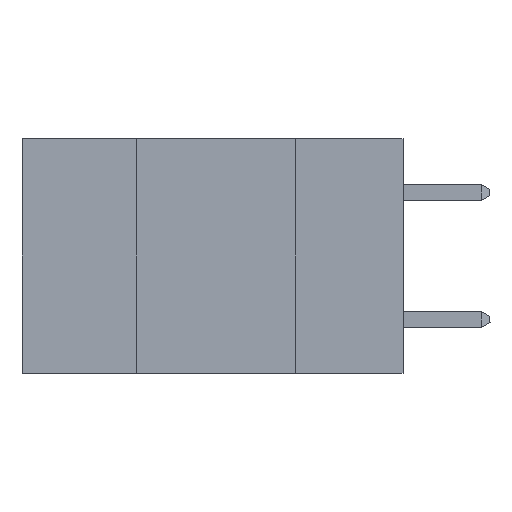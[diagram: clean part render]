
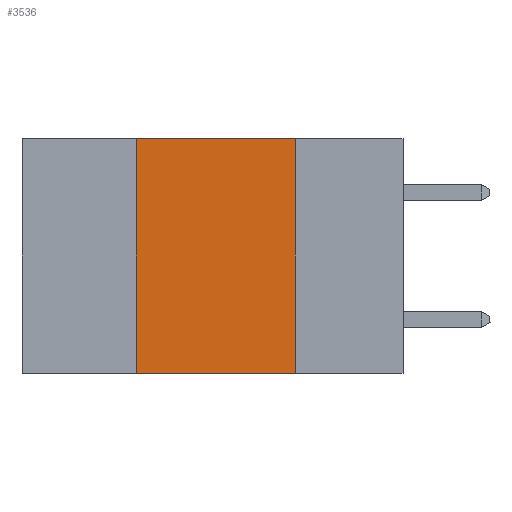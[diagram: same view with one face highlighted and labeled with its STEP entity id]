
A CAD part, left-side view. The second image highlights one B-rep face of the part: STEP entity #3536.
In plain terms, the highlighted planar face has unit normal (-1, 0, 0).
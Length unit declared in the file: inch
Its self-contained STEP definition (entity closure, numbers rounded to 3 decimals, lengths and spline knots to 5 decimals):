
#419 = CARTESIAN_POINT ( 'NONE',  ( 0., 0.42, 0. ) ) ;
#2551 = LINE ( 'NONE', #22952, #7684 ) ;
#2593 = CARTESIAN_POINT ( 'NONE',  ( 0., 0.42, 0. ) ) ;
#3536 = ADVANCED_FACE ( 'NONE', ( #6076 ), #10458, .F. ) ;
#4408 = DIRECTION ( 'NONE',  ( 1., 0., 0. ) ) ;
#4969 = VECTOR ( 'NONE', #20554, 39.37008 ) ;
#6076 = FACE_OUTER_BOUND ( 'NONE', #18062, .T. ) ;
#7684 = VECTOR ( 'NONE', #35642, 39.37008 ) ;
#10458 = PLANE ( 'NONE',  #16373 ) ;
#12220 = LINE ( 'NONE', #37124, #4969 ) ;
#13341 = EDGE_CURVE ( 'NONE', #34799, #24318, #35053, .T. ) ;
#14211 = CARTESIAN_POINT ( 'NONE',  ( 0., 0.6, 0. ) ) ;
#16373 = AXIS2_PLACEMENT_3D ( 'NONE', #14211, #4408, #37010 ) ;
#18062 = EDGE_LOOP ( 'NONE', ( #23241, #31007, #31364, #24273 ) ) ;
#20554 = DIRECTION ( 'NONE',  ( 0., -1., 0. ) ) ;
#20824 = EDGE_CURVE ( 'NONE', #35613, #22620, #31459, .T. ) ;
#22620 = VERTEX_POINT ( 'NONE', #34437 ) ;
#22952 = CARTESIAN_POINT ( 'NONE',  ( 0., 0.6, 0. ) ) ;
#23241 = ORIENTED_EDGE ( 'NONE', *, *, #20824, .F. ) ;
#24273 = ORIENTED_EDGE ( 'NONE', *, *, #30246, .T. ) ;
#24318 = VERTEX_POINT ( 'NONE', #2593 ) ;
#28190 = CARTESIAN_POINT ( 'NONE',  ( 0., 0.17, 0. ) ) ;
#30246 = EDGE_CURVE ( 'NONE', #34799, #22620, #12220, .T. ) ;
#31007 = ORIENTED_EDGE ( 'NONE', *, *, #37529, .F. ) ;
#31364 = ORIENTED_EDGE ( 'NONE', *, *, #13341, .F. ) ;
#31459 = LINE ( 'NONE', #28190, #33587 ) ;
#31875 = CARTESIAN_POINT ( 'NONE',  ( 0., 0.17, 0. ) ) ;
#32458 = VECTOR ( 'NONE', #40223, 39.37008 ) ;
#33587 = VECTOR ( 'NONE', #38366, 39.37008 ) ;
#34437 = CARTESIAN_POINT ( 'NONE',  ( 0., 0.17, -0.37 ) ) ;
#34799 = VERTEX_POINT ( 'NONE', #38170 ) ;
#35053 = LINE ( 'NONE', #419, #32458 ) ;
#35613 = VERTEX_POINT ( 'NONE', #31875 ) ;
#35642 = DIRECTION ( 'NONE',  ( 0., -1., 0. ) ) ;
#37010 = DIRECTION ( 'NONE',  ( 0., 0., -1. ) ) ;
#37124 = CARTESIAN_POINT ( 'NONE',  ( 0., 0.6, -0.37 ) ) ;
#37529 = EDGE_CURVE ( 'NONE', #24318, #35613, #2551, .T. ) ;
#38170 = CARTESIAN_POINT ( 'NONE',  ( 0., 0.42, -0.37 ) ) ;
#38366 = DIRECTION ( 'NONE',  ( 0., 0., -1. ) ) ;
#40223 = DIRECTION ( 'NONE',  ( 0., 0., 1. ) ) ;
